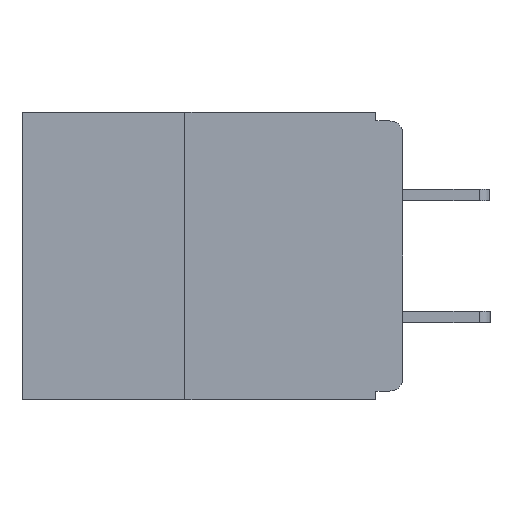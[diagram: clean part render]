
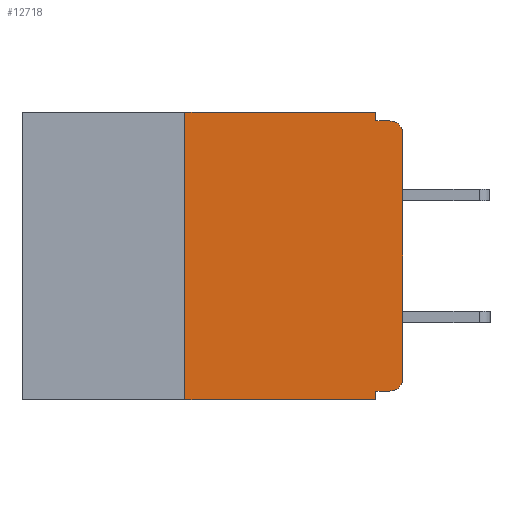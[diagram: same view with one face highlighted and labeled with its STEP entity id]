
A CAD part, left-side view. The second image highlights one B-rep face of the part: STEP entity #12718.
In plain terms, the highlighted planar face has unit normal (-1, 0, 0).
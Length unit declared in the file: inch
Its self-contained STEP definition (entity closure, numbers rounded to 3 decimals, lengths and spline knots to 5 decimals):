
#92 = CARTESIAN_POINT ( 'NONE',  ( 0., 0., -0.01 ) ) ;
#274 = ORIENTED_EDGE ( 'NONE', *, *, #1646, .F. ) ;
#319 = EDGE_CURVE ( 'NONE', #10543, #12066, #496, .T. ) ;
#409 = VERTEX_POINT ( 'NONE', #11988 ) ;
#476 = CARTESIAN_POINT ( 'NONE',  ( 0., 0.031, 0. ) ) ;
#496 = CIRCLE ( 'NONE', #9630, 0.015 ) ;
#538 = DIRECTION ( 'NONE',  ( 0., 0., -1. ) ) ;
#699 = DIRECTION ( 'NONE',  ( 0., 0., 1. ) ) ;
#874 = DIRECTION ( 'NONE',  ( 0., 0., -1. ) ) ;
#1018 = ORIENTED_EDGE ( 'NONE', *, *, #10172, .F. ) ;
#1041 = DIRECTION ( 'NONE',  ( 0., 0., -1. ) ) ;
#1164 = DIRECTION ( 'NONE',  ( -1., 0., 0. ) ) ;
#1425 = LINE ( 'NONE', #92, #4257 ) ;
#1560 = DIRECTION ( 'NONE',  ( -1., 0., 0. ) ) ;
#1646 = EDGE_CURVE ( 'NONE', #2893, #5661, #6412, .T. ) ;
#1807 = DIRECTION ( 'NONE',  ( 0., 0., 1. ) ) ;
#2674 = VERTEX_POINT ( 'NONE', #7810 ) ;
#2746 = VECTOR ( 'NONE', #12232, 39.37008 ) ;
#2893 = VERTEX_POINT ( 'NONE', #6227 ) ;
#3488 = LINE ( 'NONE', #11071, #2746 ) ;
#4257 = VECTOR ( 'NONE', #7391, 39.37008 ) ;
#4258 = ORIENTED_EDGE ( 'NONE', *, *, #319, .T. ) ;
#4303 = CARTESIAN_POINT ( 'NONE',  ( 0., 0., -0.305 ) ) ;
#4435 = CIRCLE ( 'NONE', #14142, 0.015 ) ;
#4447 = EDGE_CURVE ( 'NONE', #7374, #5824, #12952, .T. ) ;
#4511 = ORIENTED_EDGE ( 'NONE', *, *, #14088, .F. ) ;
#4595 = CARTESIAN_POINT ( 'NONE',  ( 0., 0.031, -0.32 ) ) ;
#4717 = LINE ( 'NONE', #8283, #7900 ) ;
#4885 = LINE ( 'NONE', #10211, #9778 ) ;
#5054 = CARTESIAN_POINT ( 'NONE',  ( 0., 0.031, -0.33 ) ) ;
#5332 = ORIENTED_EDGE ( 'NONE', *, *, #10546, .T. ) ;
#5528 = CARTESIAN_POINT ( 'NONE',  ( 0., 0., 0. ) ) ;
#5661 = VERTEX_POINT ( 'NONE', #11874 ) ;
#5824 = VERTEX_POINT ( 'NONE', #5054 ) ;
#5994 = VECTOR ( 'NONE', #10901, 39.37008 ) ;
#6227 = CARTESIAN_POINT ( 'NONE',  ( 0., 0.25, -0.33 ) ) ;
#6392 = ORIENTED_EDGE ( 'NONE', *, *, #12422, .F. ) ;
#6412 = LINE ( 'NONE', #7792, #12000 ) ;
#6519 = EDGE_CURVE ( 'NONE', #409, #9604, #4435, .T. ) ;
#6646 = VECTOR ( 'NONE', #9497, 39.37008 ) ;
#6728 = CARTESIAN_POINT ( 'NONE',  ( 0., 0.015, -0.32 ) ) ;
#6838 = PLANE ( 'NONE',  #7709 ) ;
#7374 = VERTEX_POINT ( 'NONE', #4595 ) ;
#7391 = DIRECTION ( 'NONE',  ( 0., -1., 0. ) ) ;
#7709 = AXIS2_PLACEMENT_3D ( 'NONE', #13942, #8115, #874 ) ;
#7792 = CARTESIAN_POINT ( 'NONE',  ( 0., 0.25, -0.33 ) ) ;
#7810 = CARTESIAN_POINT ( 'NONE',  ( 0., 0.031, -0.01 ) ) ;
#7900 = VECTOR ( 'NONE', #1041, 39.37008 ) ;
#8115 = DIRECTION ( 'NONE',  ( 1., 0., 0. ) ) ;
#8283 = CARTESIAN_POINT ( 'NONE',  ( 0., 0.031, 0. ) ) ;
#8422 = ORIENTED_EDGE ( 'NONE', *, *, #10474, .T. ) ;
#8645 = VECTOR ( 'NONE', #699, 39.37008 ) ;
#8778 = CARTESIAN_POINT ( 'NONE',  ( 0., 0.015, -0.025 ) ) ;
#9401 = LINE ( 'NONE', #5528, #8645 ) ;
#9497 = DIRECTION ( 'NONE',  ( 0., 0., -1. ) ) ;
#9548 = CARTESIAN_POINT ( 'NONE',  ( 0., 0.031, -0.33 ) ) ;
#9604 = VERTEX_POINT ( 'NONE', #14193 ) ;
#9630 = AXIS2_PLACEMENT_3D ( 'NONE', #9687, #1164, #538 ) ;
#9687 = CARTESIAN_POINT ( 'NONE',  ( 0., 0.015, -0.305 ) ) ;
#9778 = VECTOR ( 'NONE', #11374, 39.37008 ) ;
#9985 = DIRECTION ( 'NONE',  ( 0., 0., -1. ) ) ;
#10172 = EDGE_CURVE ( 'NONE', #13721, #2674, #4717, .T. ) ;
#10211 = CARTESIAN_POINT ( 'NONE',  ( 0., 0.437, -0.33 ) ) ;
#10347 = EDGE_LOOP ( 'NONE', ( #5332, #11893, #6392, #1018, #12256, #274, #8422, #13546, #4511, #4258 ) ) ;
#10474 = EDGE_CURVE ( 'NONE', #2893, #5824, #4885, .T. ) ;
#10543 = VERTEX_POINT ( 'NONE', #6728 ) ;
#10546 = EDGE_CURVE ( 'NONE', #12066, #409, #9401, .T. ) ;
#10653 = FACE_OUTER_BOUND ( 'NONE', #10347, .T. ) ;
#10901 = DIRECTION ( 'NONE',  ( 0., -1., 0. ) ) ;
#11071 = CARTESIAN_POINT ( 'NONE',  ( 0., 0., -0.32 ) ) ;
#11374 = DIRECTION ( 'NONE',  ( 0., -1., 0. ) ) ;
#11778 = EDGE_CURVE ( 'NONE', #5661, #13721, #12308, .T. ) ;
#11874 = CARTESIAN_POINT ( 'NONE',  ( 0., 0.25, 0. ) ) ;
#11893 = ORIENTED_EDGE ( 'NONE', *, *, #6519, .T. ) ;
#11988 = CARTESIAN_POINT ( 'NONE',  ( 0., 0., -0.025 ) ) ;
#12000 = VECTOR ( 'NONE', #1807, 39.37008 ) ;
#12066 = VERTEX_POINT ( 'NONE', #4303 ) ;
#12232 = DIRECTION ( 'NONE',  ( 0., 1., 0. ) ) ;
#12256 = ORIENTED_EDGE ( 'NONE', *, *, #11778, .F. ) ;
#12308 = LINE ( 'NONE', #14341, #5994 ) ;
#12422 = EDGE_CURVE ( 'NONE', #2674, #9604, #1425, .T. ) ;
#12718 = ADVANCED_FACE ( 'NONE', ( #10653 ), #6838, .F. ) ;
#12952 = LINE ( 'NONE', #9548, #6646 ) ;
#13546 = ORIENTED_EDGE ( 'NONE', *, *, #4447, .F. ) ;
#13721 = VERTEX_POINT ( 'NONE', #476 ) ;
#13942 = CARTESIAN_POINT ( 'NONE',  ( 0., 0.437, 0. ) ) ;
#14088 = EDGE_CURVE ( 'NONE', #10543, #7374, #3488, .T. ) ;
#14142 = AXIS2_PLACEMENT_3D ( 'NONE', #8778, #1560, #9985 ) ;
#14193 = CARTESIAN_POINT ( 'NONE',  ( 0., 0.015, -0.01 ) ) ;
#14341 = CARTESIAN_POINT ( 'NONE',  ( 0., 0.437, 0. ) ) ;
